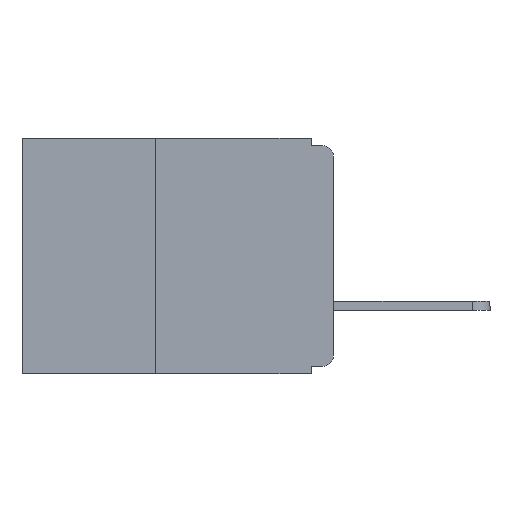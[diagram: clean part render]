
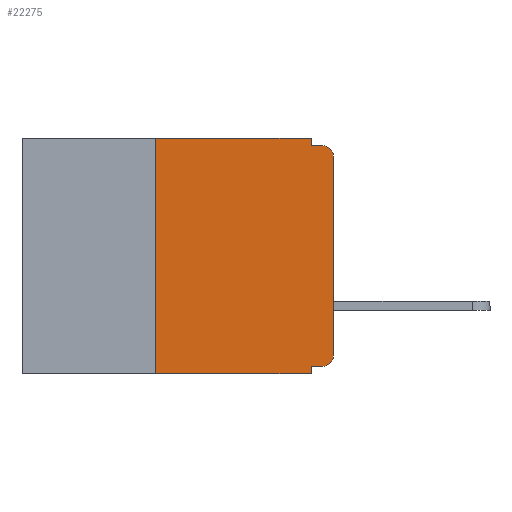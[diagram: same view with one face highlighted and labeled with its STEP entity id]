
A CAD part, left-side view. The second image highlights one B-rep face of the part: STEP entity #22275.
In plain terms, the highlighted planar face has unit normal (-1, 0, 0).
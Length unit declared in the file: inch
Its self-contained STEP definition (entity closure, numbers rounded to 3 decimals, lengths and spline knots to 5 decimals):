
#37 = VERTEX_POINT ( 'NONE', #27152 ) ;
#252 = VECTOR ( 'NONE', #31337, 39.37008 ) ;
#348 = DIRECTION ( 'NONE',  ( 0., 0., -1. ) ) ;
#653 = LINE ( 'NONE', #20132, #27183 ) ;
#1447 = VECTOR ( 'NONE', #28206, 39.37008 ) ;
#1498 = VERTEX_POINT ( 'NONE', #6085 ) ;
#1879 = EDGE_CURVE ( 'NONE', #6896, #20599, #7578, .T. ) ;
#2272 = LINE ( 'NONE', #2540, #1447 ) ;
#2475 = EDGE_CURVE ( 'NONE', #7888, #37, #26806, .T. ) ;
#2540 = CARTESIAN_POINT ( 'NONE',  ( 0., 0., -0.01 ) ) ;
#2975 = CARTESIAN_POINT ( 'NONE',  ( 0., 0.031, -0.33 ) ) ;
#3236 = VECTOR ( 'NONE', #348, 39.37008 ) ;
#3296 = ORIENTED_EDGE ( 'NONE', *, *, #11234, .T. ) ;
#3650 = ORIENTED_EDGE ( 'NONE', *, *, #31174, .T. ) ;
#3888 = EDGE_CURVE ( 'NONE', #20599, #7888, #7783, .T. ) ;
#4421 = ORIENTED_EDGE ( 'NONE', *, *, #5055, .T. ) ;
#4788 = CARTESIAN_POINT ( 'NONE',  ( 0., 0.015, -0.01 ) ) ;
#4841 = CARTESIAN_POINT ( 'NONE',  ( 0., 0.25, -0.33 ) ) ;
#4887 = EDGE_CURVE ( 'NONE', #1498, #19969, #30926, .T. ) ;
#5055 = EDGE_CURVE ( 'NONE', #19969, #29845, #18585, .T. ) ;
#6085 = CARTESIAN_POINT ( 'NONE',  ( 0., 0.015, -0.32 ) ) ;
#6512 = ORIENTED_EDGE ( 'NONE', *, *, #3888, .F. ) ;
#6544 = LINE ( 'NONE', #7492, #32886 ) ;
#6772 = PLANE ( 'NONE',  #8661 ) ;
#6896 = VERTEX_POINT ( 'NONE', #25318 ) ;
#7200 = CARTESIAN_POINT ( 'NONE',  ( 0., 0.25, 0. ) ) ;
#7492 = CARTESIAN_POINT ( 'NONE',  ( 0., 0., -0.32 ) ) ;
#7578 = LINE ( 'NONE', #4841, #25656 ) ;
#7783 = LINE ( 'NONE', #15412, #20679 ) ;
#7888 = VERTEX_POINT ( 'NONE', #21628 ) ;
#8066 = CARTESIAN_POINT ( 'NONE',  ( 0., 0.015, -0.025 ) ) ;
#8661 = AXIS2_PLACEMENT_3D ( 'NONE', #24943, #12199, #30021 ) ;
#9840 = CARTESIAN_POINT ( 'NONE',  ( 0., 0., -0.025 ) ) ;
#10680 = DIRECTION ( 'NONE',  ( 0., 0., -1. ) ) ;
#11234 = EDGE_CURVE ( 'NONE', #6896, #29690, #653, .T. ) ;
#11691 = AXIS2_PLACEMENT_3D ( 'NONE', #20867, #20831, #20803 ) ;
#11769 = VECTOR ( 'NONE', #17347, 39.37008 ) ;
#11810 = ORIENTED_EDGE ( 'NONE', *, *, #23963, .F. ) ;
#12199 = DIRECTION ( 'NONE',  ( 1., 0., 0. ) ) ;
#14362 = CARTESIAN_POINT ( 'NONE',  ( 0., 0.031, -0.33 ) ) ;
#14757 = EDGE_LOOP ( 'NONE', ( #4421, #3650, #24961, #16177, #6512, #26975, #3296, #11810, #20240, #24241 ) ) ;
#15412 = CARTESIAN_POINT ( 'NONE',  ( 0., 0.437, 0. ) ) ;
#15638 = DIRECTION ( 'NONE',  ( 0., -1., 0. ) ) ;
#16177 = ORIENTED_EDGE ( 'NONE', *, *, #2475, .F. ) ;
#16960 = LINE ( 'NONE', #2975, #3236 ) ;
#17347 = DIRECTION ( 'NONE',  ( 0., 0., 1. ) ) ;
#17535 = CARTESIAN_POINT ( 'NONE',  ( 0., 0., 0. ) ) ;
#18459 = EDGE_CURVE ( 'NONE', #37, #22978, #2272, .T. ) ;
#18585 = LINE ( 'NONE', #17535, #11769 ) ;
#19272 = VERTEX_POINT ( 'NONE', #31276 ) ;
#19293 = DIRECTION ( 'NONE',  ( 0., 0., 1. ) ) ;
#19969 = VERTEX_POINT ( 'NONE', #28984 ) ;
#20132 = CARTESIAN_POINT ( 'NONE',  ( 0., 0.437, -0.33 ) ) ;
#20240 = ORIENTED_EDGE ( 'NONE', *, *, #23035, .F. ) ;
#20599 = VERTEX_POINT ( 'NONE', #7200 ) ;
#20679 = VECTOR ( 'NONE', #15638, 39.37008 ) ;
#20803 = DIRECTION ( 'NONE',  ( 0., 0., -1. ) ) ;
#20831 = DIRECTION ( 'NONE',  ( -1., 0., 0. ) ) ;
#20867 = CARTESIAN_POINT ( 'NONE',  ( 0., 0.015, -0.305 ) ) ;
#21628 = CARTESIAN_POINT ( 'NONE',  ( 0., 0.031, 0. ) ) ;
#22275 = ADVANCED_FACE ( 'NONE', ( #28226 ), #6772, .F. ) ;
#22904 = DIRECTION ( 'NONE',  ( 0., 1., 0. ) ) ;
#22978 = VERTEX_POINT ( 'NONE', #4788 ) ;
#23035 = EDGE_CURVE ( 'NONE', #1498, #19272, #6544, .T. ) ;
#23963 = EDGE_CURVE ( 'NONE', #19272, #29690, #16960, .T. ) ;
#24241 = ORIENTED_EDGE ( 'NONE', *, *, #4887, .T. ) ;
#24943 = CARTESIAN_POINT ( 'NONE',  ( 0., 0.437, 0. ) ) ;
#24961 = ORIENTED_EDGE ( 'NONE', *, *, #18459, .F. ) ;
#25318 = CARTESIAN_POINT ( 'NONE',  ( 0., 0.25, -0.33 ) ) ;
#25656 = VECTOR ( 'NONE', #19293, 39.37008 ) ;
#26015 = DIRECTION ( 'NONE',  ( -1., 0., 0. ) ) ;
#26247 = CARTESIAN_POINT ( 'NONE',  ( 0., 0.031, 0. ) ) ;
#26425 = CIRCLE ( 'NONE', #28303, 0.015 ) ;
#26806 = LINE ( 'NONE', #26247, #252 ) ;
#26975 = ORIENTED_EDGE ( 'NONE', *, *, #1879, .F. ) ;
#27152 = CARTESIAN_POINT ( 'NONE',  ( 0., 0.031, -0.01 ) ) ;
#27183 = VECTOR ( 'NONE', #30333, 39.37008 ) ;
#28206 = DIRECTION ( 'NONE',  ( 0., -1., 0. ) ) ;
#28226 = FACE_OUTER_BOUND ( 'NONE', #14757, .T. ) ;
#28303 = AXIS2_PLACEMENT_3D ( 'NONE', #8066, #26015, #10680 ) ;
#28984 = CARTESIAN_POINT ( 'NONE',  ( 0., 0., -0.305 ) ) ;
#29690 = VERTEX_POINT ( 'NONE', #14362 ) ;
#29845 = VERTEX_POINT ( 'NONE', #9840 ) ;
#30021 = DIRECTION ( 'NONE',  ( 0., 0., -1. ) ) ;
#30333 = DIRECTION ( 'NONE',  ( 0., -1., 0. ) ) ;
#30926 = CIRCLE ( 'NONE', #11691, 0.015 ) ;
#31174 = EDGE_CURVE ( 'NONE', #29845, #22978, #26425, .T. ) ;
#31276 = CARTESIAN_POINT ( 'NONE',  ( 0., 0.031, -0.32 ) ) ;
#31337 = DIRECTION ( 'NONE',  ( 0., 0., -1. ) ) ;
#32886 = VECTOR ( 'NONE', #22904, 39.37008 ) ;
